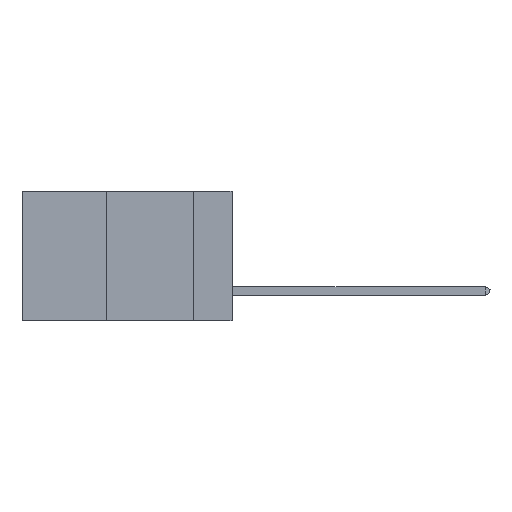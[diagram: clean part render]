
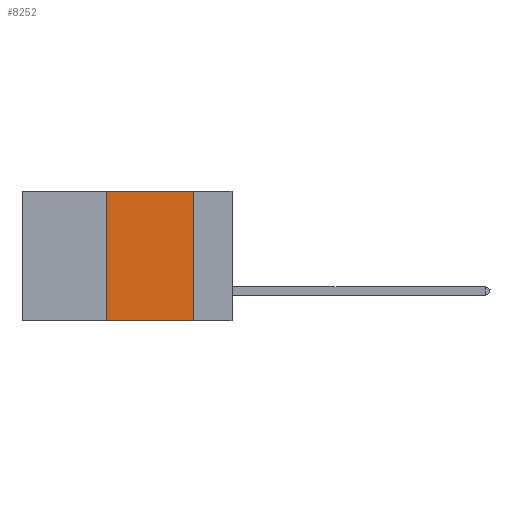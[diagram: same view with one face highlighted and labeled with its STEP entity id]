
A CAD part, left-side view. The second image highlights one B-rep face of the part: STEP entity #8252.
In plain terms, the highlighted planar face has unit normal (-1, 0, 0).
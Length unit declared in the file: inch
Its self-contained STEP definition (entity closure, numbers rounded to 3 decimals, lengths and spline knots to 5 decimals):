
#988 = ORIENTED_EDGE ( 'NONE', *, *, #4309, .T. ) ;
#2331 = ORIENTED_EDGE ( 'NONE', *, *, #19134, .F. ) ;
#4246 = LINE ( 'NONE', #31480, #30018 ) ;
#4309 = EDGE_CURVE ( 'NONE', #9235, #33232, #15762, .T. ) ;
#5516 = CARTESIAN_POINT ( 'NONE',  ( 0., 0.11, -0.37 ) ) ;
#5568 = CARTESIAN_POINT ( 'NONE',  ( 0., 0.11, 0. ) ) ;
#6130 = CARTESIAN_POINT ( 'NONE',  ( 0., 0.6, 0. ) ) ;
#7587 = CARTESIAN_POINT ( 'NONE',  ( 0., 0.36, 0. ) ) ;
#8252 = ADVANCED_FACE ( 'NONE', ( #14323 ), #16936, .F. ) ;
#8792 = VECTOR ( 'NONE', #16394, 39.37008 ) ;
#9235 = VERTEX_POINT ( 'NONE', #13731 ) ;
#9613 = ORIENTED_EDGE ( 'NONE', *, *, #12324, .F. ) ;
#10970 = EDGE_LOOP ( 'NONE', ( #2331, #9613, #15373, #988 ) ) ;
#12241 = DIRECTION ( 'NONE',  ( 0., -1., 0. ) ) ;
#12324 = EDGE_CURVE ( 'NONE', #29552, #19661, #30592, .T. ) ;
#13731 = CARTESIAN_POINT ( 'NONE',  ( 0., 0.36, -0.37 ) ) ;
#14323 = FACE_OUTER_BOUND ( 'NONE', #10970, .T. ) ;
#15373 = ORIENTED_EDGE ( 'NONE', *, *, #24431, .F. ) ;
#15486 = LINE ( 'NONE', #22310, #29225 ) ;
#15762 = LINE ( 'NONE', #19586, #23498 ) ;
#16297 = DIRECTION ( 'NONE',  ( 0., 0., -1. ) ) ;
#16394 = DIRECTION ( 'NONE',  ( 0., -1., 0. ) ) ;
#16936 = PLANE ( 'NONE',  #21122 ) ;
#19062 = DIRECTION ( 'NONE',  ( 1., 0., 0. ) ) ;
#19134 = EDGE_CURVE ( 'NONE', #19661, #33232, #4246, .T. ) ;
#19586 = CARTESIAN_POINT ( 'NONE',  ( 0., 0.6, -0.37 ) ) ;
#19661 = VERTEX_POINT ( 'NONE', #5568 ) ;
#21122 = AXIS2_PLACEMENT_3D ( 'NONE', #29884, #19062, #31903 ) ;
#22310 = CARTESIAN_POINT ( 'NONE',  ( 0., 0.36, 0. ) ) ;
#23498 = VECTOR ( 'NONE', #12241, 39.37008 ) ;
#24431 = EDGE_CURVE ( 'NONE', #9235, #29552, #15486, .T. ) ;
#29225 = VECTOR ( 'NONE', #32422, 39.37008 ) ;
#29552 = VERTEX_POINT ( 'NONE', #7587 ) ;
#29884 = CARTESIAN_POINT ( 'NONE',  ( 0., 0.6, 0. ) ) ;
#30018 = VECTOR ( 'NONE', #16297, 39.37008 ) ;
#30592 = LINE ( 'NONE', #6130, #8792 ) ;
#31480 = CARTESIAN_POINT ( 'NONE',  ( 0., 0.11, 0. ) ) ;
#31903 = DIRECTION ( 'NONE',  ( 0., 0., -1. ) ) ;
#32422 = DIRECTION ( 'NONE',  ( 0., 0., 1. ) ) ;
#33232 = VERTEX_POINT ( 'NONE', #5516 ) ;
